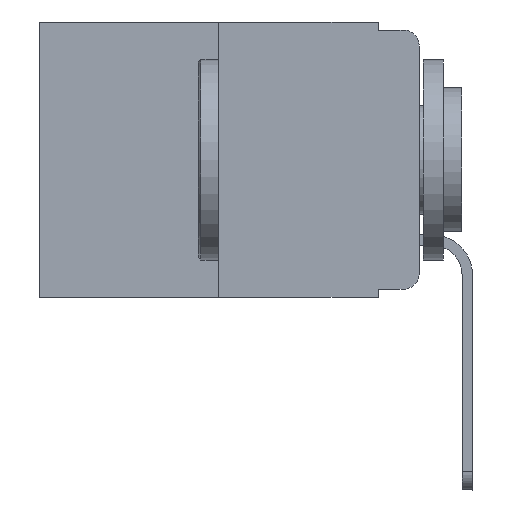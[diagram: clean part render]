
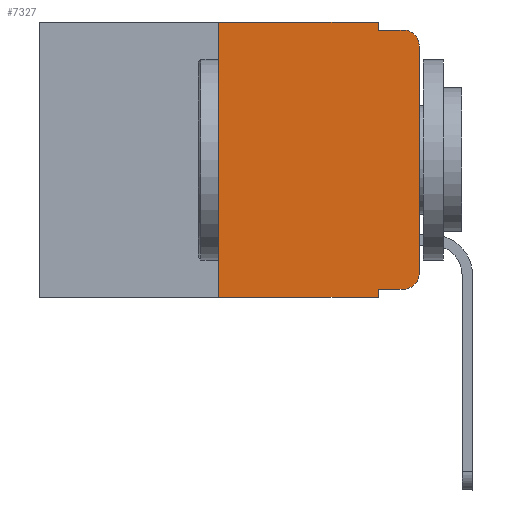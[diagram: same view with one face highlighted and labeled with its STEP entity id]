
A CAD part, left-side view. The second image highlights one B-rep face of the part: STEP entity #7327.
In plain terms, the highlighted planar face has unit normal (-1, 0, 0).
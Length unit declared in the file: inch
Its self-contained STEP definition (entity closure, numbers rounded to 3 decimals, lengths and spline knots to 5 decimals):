
#536 = DIRECTION ( 'NONE',  ( 0., -1., 0. ) ) ;
#670 = AXIS2_PLACEMENT_3D ( 'NONE', #4641, #8390, #20570 ) ;
#835 = VERTEX_POINT ( 'NONE', #5131 ) ;
#1160 = CARTESIAN_POINT ( 'NONE',  ( 0., 0.25, -0.343 ) ) ;
#1229 = AXIS2_PLACEMENT_3D ( 'NONE', #10430, #4752, #8619 ) ;
#1283 = LINE ( 'NONE', #20390, #20112 ) ;
#2074 = CARTESIAN_POINT ( 'NONE',  ( 0., 0., -0.313 ) ) ;
#2384 = VERTEX_POINT ( 'NONE', #9729 ) ;
#2743 = ORIENTED_EDGE ( 'NONE', *, *, #4057, .F. ) ;
#2762 = EDGE_LOOP ( 'NONE', ( #13988, #10371, #7101, #8199, #5860, #5077, #19619, #2743, #7719, #11809 ) ) ;
#2888 = LINE ( 'NONE', #16110, #14789 ) ;
#2945 = CIRCLE ( 'NONE', #14212, 0.02 ) ;
#3039 = PLANE ( 'NONE',  #1229 ) ;
#3053 = DIRECTION ( 'NONE',  ( 0., -1., 0. ) ) ;
#3231 = EDGE_CURVE ( 'NONE', #14487, #15822, #6125, .T. ) ;
#3854 = EDGE_CURVE ( 'NONE', #2384, #16976, #20986, .T. ) ;
#3860 = CARTESIAN_POINT ( 'NONE',  ( 0., 0., -0.03 ) ) ;
#3896 = CARTESIAN_POINT ( 'NONE',  ( 0., 0.051, -0.01 ) ) ;
#4057 = EDGE_CURVE ( 'NONE', #835, #13616, #1283, .T. ) ;
#4118 = DIRECTION ( 'NONE',  ( 0., 0., -1. ) ) ;
#4339 = DIRECTION ( 'NONE',  ( -1., 0., 0. ) ) ;
#4641 = CARTESIAN_POINT ( 'NONE',  ( 0., 0.02, -0.03 ) ) ;
#4752 = DIRECTION ( 'NONE',  ( 1., 0., 0. ) ) ;
#4958 = CARTESIAN_POINT ( 'NONE',  ( 0., 0.473, 0. ) ) ;
#5077 = ORIENTED_EDGE ( 'NONE', *, *, #14051, .F. ) ;
#5131 = CARTESIAN_POINT ( 'NONE',  ( 0., 0.051, -0.333 ) ) ;
#5304 = VERTEX_POINT ( 'NONE', #15903 ) ;
#5692 = DIRECTION ( 'NONE',  ( 0., -1., 0. ) ) ;
#5703 = LINE ( 'NONE', #14855, #13571 ) ;
#5718 = CARTESIAN_POINT ( 'NONE',  ( 0., 0.25, 0. ) ) ;
#5860 = ORIENTED_EDGE ( 'NONE', *, *, #3854, .F. ) ;
#6125 = CIRCLE ( 'NONE', #670, 0.02 ) ;
#7101 = ORIENTED_EDGE ( 'NONE', *, *, #13494, .F. ) ;
#7183 = EDGE_CURVE ( 'NONE', #16976, #21660, #5703, .T. ) ;
#7327 = ADVANCED_FACE ( 'NONE', ( #18610 ), #3039, .F. ) ;
#7521 = DIRECTION ( 'NONE',  ( 0., 0., 1. ) ) ;
#7719 = ORIENTED_EDGE ( 'NONE', *, *, #14444, .T. ) ;
#8109 = DIRECTION ( 'NONE',  ( 0., 0., -1. ) ) ;
#8199 = ORIENTED_EDGE ( 'NONE', *, *, #7183, .F. ) ;
#8390 = DIRECTION ( 'NONE',  ( -1., 0., 0. ) ) ;
#8619 = DIRECTION ( 'NONE',  ( 0., 0., -1. ) ) ;
#8886 = CARTESIAN_POINT ( 'NONE',  ( 0., 0.02, -0.01 ) ) ;
#9488 = VECTOR ( 'NONE', #7521, 39.37008 ) ;
#9729 = CARTESIAN_POINT ( 'NONE',  ( 0., 0.25, 0. ) ) ;
#10371 = ORIENTED_EDGE ( 'NONE', *, *, #3231, .T. ) ;
#10430 = CARTESIAN_POINT ( 'NONE',  ( 0., 0.473, 0. ) ) ;
#10826 = VECTOR ( 'NONE', #11490, 39.37008 ) ;
#11490 = DIRECTION ( 'NONE',  ( 0., 0., 1. ) ) ;
#11809 = ORIENTED_EDGE ( 'NONE', *, *, #14184, .T. ) ;
#12367 = CARTESIAN_POINT ( 'NONE',  ( 0., 0.051, -0.343 ) ) ;
#12515 = LINE ( 'NONE', #19211, #21863 ) ;
#13191 = LINE ( 'NONE', #20132, #10826 ) ;
#13494 = EDGE_CURVE ( 'NONE', #21660, #15822, #17142, .T. ) ;
#13571 = VECTOR ( 'NONE', #17845, 39.37008 ) ;
#13616 = VERTEX_POINT ( 'NONE', #12367 ) ;
#13988 = ORIENTED_EDGE ( 'NONE', *, *, #22356, .T. ) ;
#14025 = VERTEX_POINT ( 'NONE', #2074 ) ;
#14051 = EDGE_CURVE ( 'NONE', #20443, #2384, #17865, .T. ) ;
#14184 = EDGE_CURVE ( 'NONE', #5304, #14025, #2945, .T. ) ;
#14212 = AXIS2_PLACEMENT_3D ( 'NONE', #17973, #4339, #4118 ) ;
#14444 = EDGE_CURVE ( 'NONE', #835, #5304, #12515, .T. ) ;
#14487 = VERTEX_POINT ( 'NONE', #3860 ) ;
#14789 = VECTOR ( 'NONE', #536, 39.37008 ) ;
#14855 = CARTESIAN_POINT ( 'NONE',  ( 0., 0.051, 0. ) ) ;
#15262 = VECTOR ( 'NONE', #3053, 39.37008 ) ;
#15822 = VERTEX_POINT ( 'NONE', #8886 ) ;
#15903 = CARTESIAN_POINT ( 'NONE',  ( 0., 0.02, -0.333 ) ) ;
#16110 = CARTESIAN_POINT ( 'NONE',  ( 0., 0.473, -0.343 ) ) ;
#16870 = CARTESIAN_POINT ( 'NONE',  ( 0., 0.051, 0. ) ) ;
#16976 = VERTEX_POINT ( 'NONE', #16870 ) ;
#17142 = LINE ( 'NONE', #22294, #15262 ) ;
#17845 = DIRECTION ( 'NONE',  ( 0., 0., -1. ) ) ;
#17865 = LINE ( 'NONE', #5718, #9488 ) ;
#17973 = CARTESIAN_POINT ( 'NONE',  ( 0., 0.02, -0.313 ) ) ;
#18610 = FACE_OUTER_BOUND ( 'NONE', #2762, .T. ) ;
#19211 = CARTESIAN_POINT ( 'NONE',  ( 0., 0.051, -0.333 ) ) ;
#19619 = ORIENTED_EDGE ( 'NONE', *, *, #21448, .T. ) ;
#20112 = VECTOR ( 'NONE', #8109, 39.37008 ) ;
#20132 = CARTESIAN_POINT ( 'NONE',  ( 0., 0., 0. ) ) ;
#20390 = CARTESIAN_POINT ( 'NONE',  ( 0., 0.051, 0. ) ) ;
#20443 = VERTEX_POINT ( 'NONE', #1160 ) ;
#20570 = DIRECTION ( 'NONE',  ( 0., 0., -1. ) ) ;
#20767 = DIRECTION ( 'NONE',  ( 0., -1., 0. ) ) ;
#20986 = LINE ( 'NONE', #4958, #21189 ) ;
#21189 = VECTOR ( 'NONE', #20767, 39.37008 ) ;
#21448 = EDGE_CURVE ( 'NONE', #20443, #13616, #2888, .T. ) ;
#21660 = VERTEX_POINT ( 'NONE', #3896 ) ;
#21863 = VECTOR ( 'NONE', #5692, 39.37008 ) ;
#22294 = CARTESIAN_POINT ( 'NONE',  ( 0., 0.051, -0.01 ) ) ;
#22356 = EDGE_CURVE ( 'NONE', #14025, #14487, #13191, .T. ) ;
